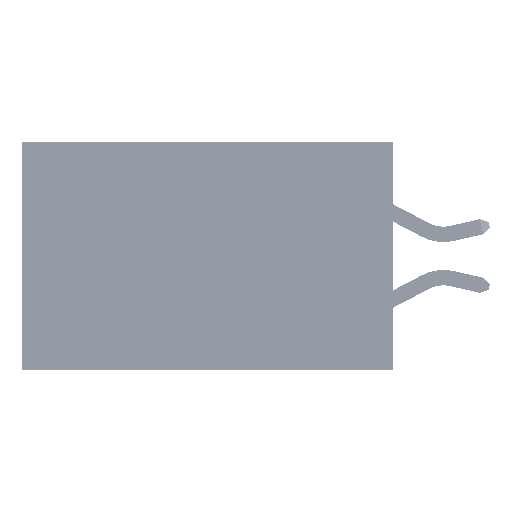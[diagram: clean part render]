
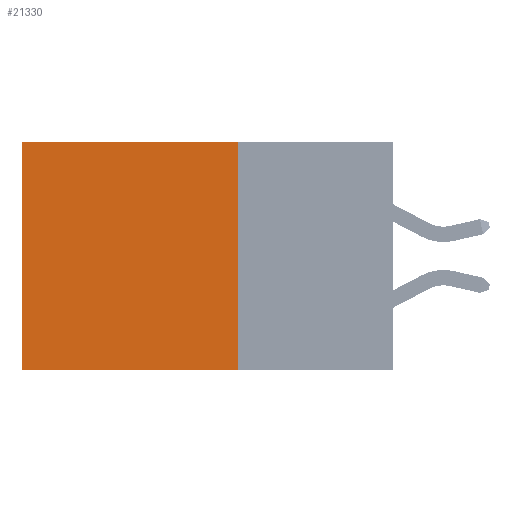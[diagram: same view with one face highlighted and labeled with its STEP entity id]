
A CAD part, left-side view. The second image highlights one B-rep face of the part: STEP entity #21330.
In plain terms, the highlighted planar face has unit normal (-1, 0, 0).
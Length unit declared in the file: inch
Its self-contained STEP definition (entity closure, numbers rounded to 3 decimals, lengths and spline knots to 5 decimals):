
#412 = PLANE ( 'NONE',  #5474 ) ;
#2349 = LINE ( 'NONE', #39844, #12620 ) ;
#4684 = EDGE_CURVE ( 'NONE', #40790, #9139, #42666, .T. ) ;
#5474 = AXIS2_PLACEMENT_3D ( 'NONE', #8150, #12031, #38645 ) ;
#5725 = VECTOR ( 'NONE', #13471, 39.37008 ) ;
#6383 = CARTESIAN_POINT ( 'NONE',  ( 0.2875, 0.25, 0. ) ) ;
#6699 = CARTESIAN_POINT ( 'NONE',  ( 0.2875, 0.6, -0.37 ) ) ;
#7114 = DIRECTION ( 'NONE',  ( 0., 1., 0. ) ) ;
#8150 = CARTESIAN_POINT ( 'NONE',  ( 0.2875, 0.25, 0. ) ) ;
#9139 = VERTEX_POINT ( 'NONE', #45771 ) ;
#9556 = CARTESIAN_POINT ( 'NONE',  ( 0.2875, 0.25, -0.37 ) ) ;
#11510 = EDGE_LOOP ( 'NONE', ( #44187, #18433, #35589, #44140 ) ) ;
#12031 = DIRECTION ( 'NONE',  ( 1., 0., 0. ) ) ;
#12620 = VECTOR ( 'NONE', #13286, 39.37008 ) ;
#13286 = DIRECTION ( 'NONE',  ( 0., 0., -1. ) ) ;
#13471 = DIRECTION ( 'NONE',  ( 0., 1., 0. ) ) ;
#18433 = ORIENTED_EDGE ( 'NONE', *, *, #34391, .F. ) ;
#18532 = CARTESIAN_POINT ( 'NONE',  ( 0.2875, 0.25, 0. ) ) ;
#20426 = EDGE_CURVE ( 'NONE', #9139, #25638, #21244, .T. ) ;
#21244 = LINE ( 'NONE', #37393, #26594 ) ;
#21330 = ADVANCED_FACE ( 'NONE', ( #26500 ), #412, .F. ) ;
#21648 = CARTESIAN_POINT ( 'NONE',  ( 0.2875, 0.25, -0.37 ) ) ;
#22543 = VECTOR ( 'NONE', #7114, 39.37008 ) ;
#25571 = VERTEX_POINT ( 'NONE', #21648 ) ;
#25638 = VERTEX_POINT ( 'NONE', #6699 ) ;
#26143 = DIRECTION ( 'NONE',  ( 0., 0., -1. ) ) ;
#26500 = FACE_OUTER_BOUND ( 'NONE', #11510, .T. ) ;
#26594 = VECTOR ( 'NONE', #26143, 39.37008 ) ;
#28101 = EDGE_CURVE ( 'NONE', #40790, #25571, #2349, .T. ) ;
#34391 = EDGE_CURVE ( 'NONE', #25571, #25638, #46217, .T. ) ;
#35589 = ORIENTED_EDGE ( 'NONE', *, *, #28101, .F. ) ;
#37393 = CARTESIAN_POINT ( 'NONE',  ( 0.2875, 0.6, 0. ) ) ;
#38645 = DIRECTION ( 'NONE',  ( 0., 0., -1. ) ) ;
#39844 = CARTESIAN_POINT ( 'NONE',  ( 0.2875, 0.25, 0. ) ) ;
#40790 = VERTEX_POINT ( 'NONE', #6383 ) ;
#42666 = LINE ( 'NONE', #18532, #22543 ) ;
#44140 = ORIENTED_EDGE ( 'NONE', *, *, #4684, .T. ) ;
#44187 = ORIENTED_EDGE ( 'NONE', *, *, #20426, .T. ) ;
#45771 = CARTESIAN_POINT ( 'NONE',  ( 0.2875, 0.6, 0. ) ) ;
#46217 = LINE ( 'NONE', #9556, #5725 ) ;
